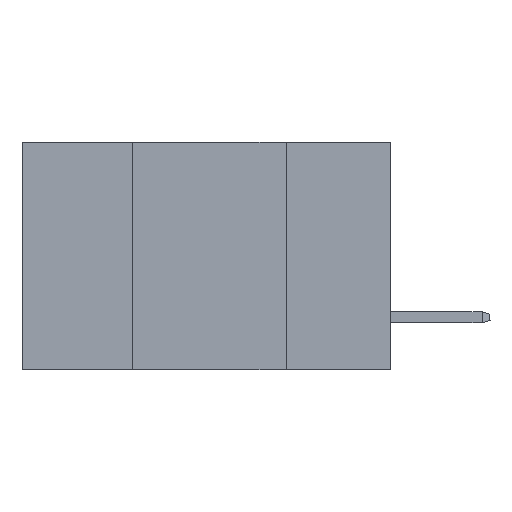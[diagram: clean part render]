
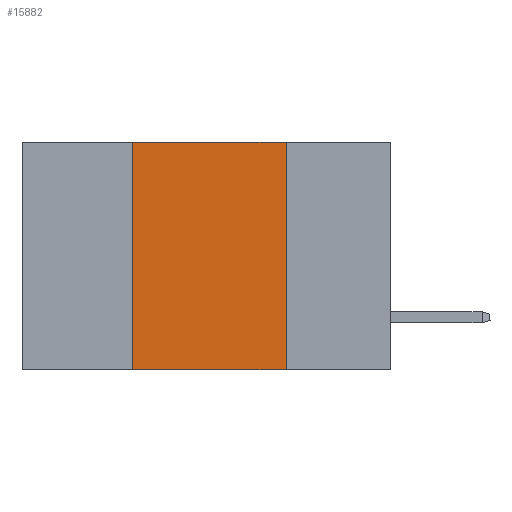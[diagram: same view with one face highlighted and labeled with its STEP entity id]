
A CAD part, left-side view. The second image highlights one B-rep face of the part: STEP entity #15882.
In plain terms, the highlighted planar face has unit normal (-1, 0, 0).
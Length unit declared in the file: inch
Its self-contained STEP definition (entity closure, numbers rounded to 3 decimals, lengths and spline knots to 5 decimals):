
#765 = CARTESIAN_POINT ( 'NONE',  ( 0., 0.42, -0.37 ) ) ;
#3083 = LINE ( 'NONE', #17667, #20455 ) ;
#4944 = AXIS2_PLACEMENT_3D ( 'NONE', #28182, #21375, #14778 ) ;
#5761 = PLANE ( 'NONE',  #4944 ) ;
#6828 = EDGE_LOOP ( 'NONE', ( #18347, #13169, #9374, #18240 ) ) ;
#7384 = VECTOR ( 'NONE', #20088, 39.37008 ) ;
#8435 = DIRECTION ( 'NONE',  ( 0., -1., 0. ) ) ;
#9374 = ORIENTED_EDGE ( 'NONE', *, *, #27126, .F. ) ;
#10119 = VERTEX_POINT ( 'NONE', #12665 ) ;
#10960 = LINE ( 'NONE', #11535, #16539 ) ;
#11535 = CARTESIAN_POINT ( 'NONE',  ( 0., 0.6, -0.37 ) ) ;
#12665 = CARTESIAN_POINT ( 'NONE',  ( 0., 0.17, 0. ) ) ;
#13169 = ORIENTED_EDGE ( 'NONE', *, *, #25008, .F. ) ;
#13899 = CARTESIAN_POINT ( 'NONE',  ( 0., 0.17, -0.37 ) ) ;
#14040 = DIRECTION ( 'NONE',  ( 0., -1., 0. ) ) ;
#14495 = EDGE_CURVE ( 'NONE', #10119, #28117, #22640, .T. ) ;
#14778 = DIRECTION ( 'NONE',  ( 0., 0., -1. ) ) ;
#15681 = VERTEX_POINT ( 'NONE', #16010 ) ;
#15882 = ADVANCED_FACE ( 'NONE', ( #19426 ), #5761, .F. ) ;
#16010 = CARTESIAN_POINT ( 'NONE',  ( 0., 0.42, 0. ) ) ;
#16119 = VERTEX_POINT ( 'NONE', #765 ) ;
#16539 = VECTOR ( 'NONE', #14040, 39.37008 ) ;
#17667 = CARTESIAN_POINT ( 'NONE',  ( 0., 0.6, 0. ) ) ;
#18240 = ORIENTED_EDGE ( 'NONE', *, *, #24418, .T. ) ;
#18347 = ORIENTED_EDGE ( 'NONE', *, *, #14495, .F. ) ;
#19426 = FACE_OUTER_BOUND ( 'NONE', #6828, .T. ) ;
#20088 = DIRECTION ( 'NONE',  ( 0., 0., 1. ) ) ;
#20455 = VECTOR ( 'NONE', #8435, 39.37008 ) ;
#21375 = DIRECTION ( 'NONE',  ( 1., 0., 0. ) ) ;
#22640 = LINE ( 'NONE', #23456, #27155 ) ;
#23456 = CARTESIAN_POINT ( 'NONE',  ( 0., 0.17, 0. ) ) ;
#24418 = EDGE_CURVE ( 'NONE', #16119, #28117, #10960, .T. ) ;
#24475 = CARTESIAN_POINT ( 'NONE',  ( 0., 0.42, 0. ) ) ;
#24713 = LINE ( 'NONE', #24475, #7384 ) ;
#25008 = EDGE_CURVE ( 'NONE', #15681, #10119, #3083, .T. ) ;
#25769 = DIRECTION ( 'NONE',  ( 0., 0., -1. ) ) ;
#27126 = EDGE_CURVE ( 'NONE', #16119, #15681, #24713, .T. ) ;
#27155 = VECTOR ( 'NONE', #25769, 39.37008 ) ;
#28117 = VERTEX_POINT ( 'NONE', #13899 ) ;
#28182 = CARTESIAN_POINT ( 'NONE',  ( 0., 0.6, 0. ) ) ;
